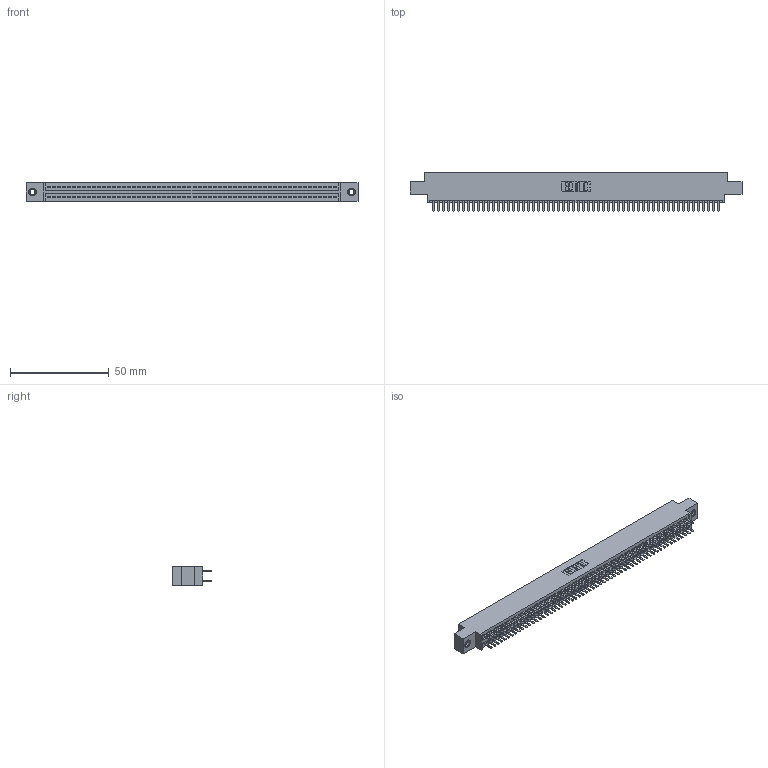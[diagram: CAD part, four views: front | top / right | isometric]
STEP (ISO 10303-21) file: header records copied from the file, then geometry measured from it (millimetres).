
FILE_DESCRIPTION (( 'STEP AP203' ), '1' );
FILE_NAME ('395-116-520-807.STEP', '2018-12-01T21:18:31', ( '' ), ( '' ), 'SwSTEP 2.0', 'SolidWorks 2016', '' );
FILE_SCHEMA (( 'CONFIG_CONTROL_DESIGN' ));
Length unit declared in the file: inch
Products named in the file (4): 345 Part_0.170 Offset - 0.156 Dia-TI; 395-116-520-807; 345-250-001_345-250-005-103; 345-292-001_345-293-120
Assembly tree (119 placements, depth 2):
  395-116-520-807
    345 Part_0.170 Offset - 0.156 Dia-TI
    345-292-001_345-293-120  x116
    345-250-001_345-250-005-103  x2
Bounding box: 168.53 x 19.68 x 9.4 mm (x, y, z)
Volume: 16341.7 mm3; surface area: 24528.6 mm2
Topology: 119 solids, 119 shells, 6454 faces, 18701 edges, 12150 vertices
Faces by surface type: plane 4176, cylinder 2262, cone 12, torus 4
Entity records: 44786 total; most frequent: CARTESIAN_POINT 7487, ORIENTED_EDGE 7402, DIRECTION 6595, EDGE_CURVE 3701, VECTOR 3313, LINE 3313, VERTEX_POINT 2460, AXIS2_PLACEMENT_3D 1641
